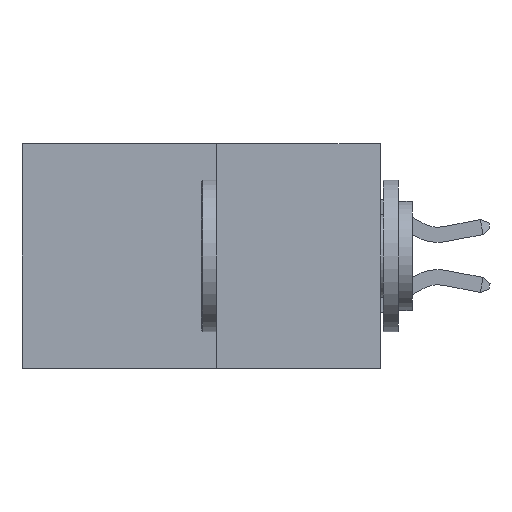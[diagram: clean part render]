
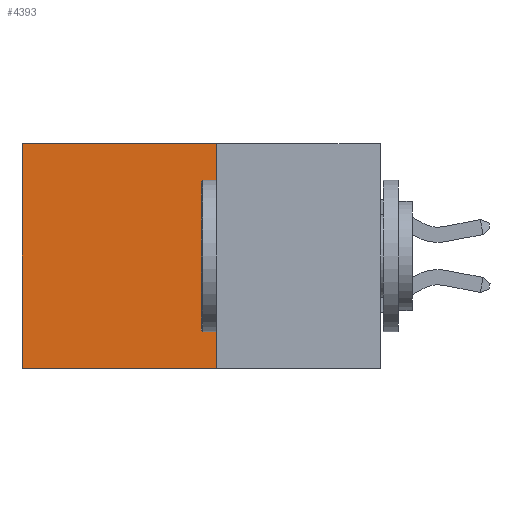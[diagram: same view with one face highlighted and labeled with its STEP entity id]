
A CAD part, left-side view. The second image highlights one B-rep face of the part: STEP entity #4393.
In plain terms, the highlighted planar face has unit normal (-1, 0, 0).
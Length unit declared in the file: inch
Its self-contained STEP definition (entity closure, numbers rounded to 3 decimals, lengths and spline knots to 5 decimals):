
#166 = CARTESIAN_POINT ( 'NONE',  ( 0.277, 0.27, -0.37 ) ) ;
#889 = DIRECTION ( 'NONE',  ( 0., 1., 0. ) ) ;
#1113 = AXIS2_PLACEMENT_3D ( 'NONE', #6324, #6313, #6301 ) ;
#1127 = VECTOR ( 'NONE', #889, 39.37008 ) ;
#1210 = ORIENTED_EDGE ( 'NONE', *, *, #2432, .T. ) ;
#1597 = EDGE_CURVE ( 'NONE', #2172, #8093, #3285, .T. ) ;
#2016 = EDGE_CURVE ( 'NONE', #6159, #3730, #6814, .T. ) ;
#2172 = VERTEX_POINT ( 'NONE', #4392 ) ;
#2375 = LINE ( 'NONE', #166, #1127 ) ;
#2432 = EDGE_CURVE ( 'NONE', #2172, #6159, #8923, .T. ) ;
#2558 = EDGE_LOOP ( 'NONE', ( #5128, #2831, #3239, #1210 ) ) ;
#2783 = VECTOR ( 'NONE', #5970, 39.37008 ) ;
#2831 = ORIENTED_EDGE ( 'NONE', *, *, #6144, .F. ) ;
#2941 = DIRECTION ( 'NONE',  ( 0., 1., 0. ) ) ;
#3239 = ORIENTED_EDGE ( 'NONE', *, *, #1597, .F. ) ;
#3285 = LINE ( 'NONE', #6754, #8786 ) ;
#3730 = VERTEX_POINT ( 'NONE', #7689 ) ;
#4392 = CARTESIAN_POINT ( 'NONE',  ( 0.277, 0.27, 0. ) ) ;
#4393 = ADVANCED_FACE ( 'NONE', ( #6553 ), #6345, .F. ) ;
#5128 = ORIENTED_EDGE ( 'NONE', *, *, #2016, .T. ) ;
#5401 = DIRECTION ( 'NONE',  ( 0., 0., -1. ) ) ;
#5893 = CARTESIAN_POINT ( 'NONE',  ( 0.277, 0.59, 0. ) ) ;
#5970 = DIRECTION ( 'NONE',  ( 0., 0., -1. ) ) ;
#6144 = EDGE_CURVE ( 'NONE', #8093, #3730, #2375, .T. ) ;
#6159 = VERTEX_POINT ( 'NONE', #5893 ) ;
#6301 = DIRECTION ( 'NONE',  ( 0., 0., -1. ) ) ;
#6313 = DIRECTION ( 'NONE',  ( 1., 0., 0. ) ) ;
#6324 = CARTESIAN_POINT ( 'NONE',  ( 0.277, 0.27, -0.37 ) ) ;
#6345 = PLANE ( 'NONE',  #1113 ) ;
#6553 = FACE_OUTER_BOUND ( 'NONE', #2558, .T. ) ;
#6754 = CARTESIAN_POINT ( 'NONE',  ( 0.277, 0.27, -0.37 ) ) ;
#6814 = LINE ( 'NONE', #9209, #2783 ) ;
#7681 = CARTESIAN_POINT ( 'NONE',  ( 0.277, 0.27, 0. ) ) ;
#7689 = CARTESIAN_POINT ( 'NONE',  ( 0.277, 0.59, -0.37 ) ) ;
#8093 = VERTEX_POINT ( 'NONE', #8557 ) ;
#8557 = CARTESIAN_POINT ( 'NONE',  ( 0.277, 0.27, -0.37 ) ) ;
#8716 = VECTOR ( 'NONE', #2941, 39.37008 ) ;
#8786 = VECTOR ( 'NONE', #5401, 39.37008 ) ;
#8923 = LINE ( 'NONE', #7681, #8716 ) ;
#9209 = CARTESIAN_POINT ( 'NONE',  ( 0.277, 0.59, -0.37 ) ) ;
